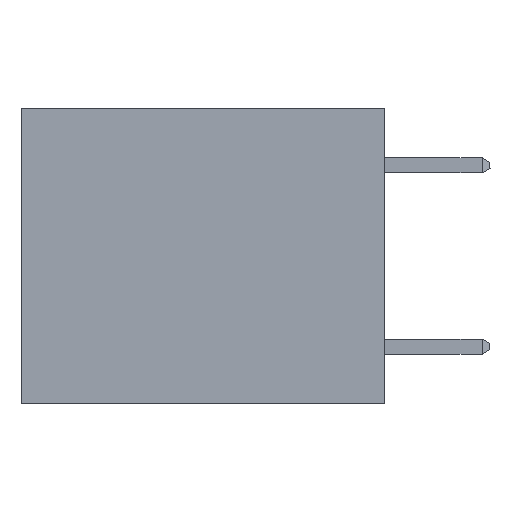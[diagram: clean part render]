
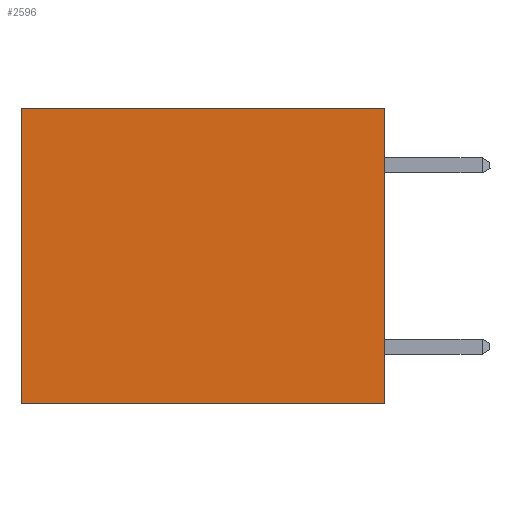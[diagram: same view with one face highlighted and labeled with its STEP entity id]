
A CAD part, left-side view. The second image highlights one B-rep face of the part: STEP entity #2596.
In plain terms, the highlighted planar face has unit normal (-1, 0, 0).
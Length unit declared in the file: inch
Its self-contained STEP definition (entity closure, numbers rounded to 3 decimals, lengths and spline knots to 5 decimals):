
#503 = LINE ( 'NONE', #11311, #14842 ) ;
#2243 = EDGE_LOOP ( 'NONE', ( #10357, #7901, #16710, #20485 ) ) ;
#2596 = ADVANCED_FACE ( 'NONE', ( #7698 ), #6340, .F. ) ;
#2666 = VERTEX_POINT ( 'NONE', #19860 ) ;
#2675 = DIRECTION ( 'NONE',  ( 1., 0., 0. ) ) ;
#3147 = LINE ( 'NONE', #20656, #10557 ) ;
#4397 = LINE ( 'NONE', #13259, #13027 ) ;
#4761 = EDGE_CURVE ( 'NONE', #2666, #6212, #4397, .T. ) ;
#5041 = CARTESIAN_POINT ( 'NONE',  ( 0.3165, 0.6, -0.49 ) ) ;
#6212 = VERTEX_POINT ( 'NONE', #5041 ) ;
#6340 = PLANE ( 'NONE',  #24676 ) ;
#7698 = FACE_OUTER_BOUND ( 'NONE', #2243, .T. ) ;
#7901 = ORIENTED_EDGE ( 'NONE', *, *, #15280, .F. ) ;
#8558 = VERTEX_POINT ( 'NONE', #13615 ) ;
#9403 = DIRECTION ( 'NONE',  ( 0., 0., -1. ) ) ;
#9563 = CARTESIAN_POINT ( 'NONE',  ( 0.3165, 0., -0.49 ) ) ;
#10130 = CARTESIAN_POINT ( 'NONE',  ( 0.3165, 0., -0.49 ) ) ;
#10357 = ORIENTED_EDGE ( 'NONE', *, *, #4761, .T. ) ;
#10557 = VECTOR ( 'NONE', #14275, 39.37008 ) ;
#11311 = CARTESIAN_POINT ( 'NONE',  ( 0.3165, 0., 0. ) ) ;
#11955 = EDGE_CURVE ( 'NONE', #8558, #18296, #21209, .T. ) ;
#12585 = CARTESIAN_POINT ( 'NONE',  ( 0.3165, 0., -0.49 ) ) ;
#13027 = VECTOR ( 'NONE', #23129, 39.37008 ) ;
#13259 = CARTESIAN_POINT ( 'NONE',  ( 0.3165, 0.6, -0.49 ) ) ;
#13426 = EDGE_CURVE ( 'NONE', #8558, #2666, #503, .T. ) ;
#13543 = DIRECTION ( 'NONE',  ( 0., 1., 0. ) ) ;
#13615 = CARTESIAN_POINT ( 'NONE',  ( 0.3165, 0., 0. ) ) ;
#14275 = DIRECTION ( 'NONE',  ( 0., 1., 0. ) ) ;
#14842 = VECTOR ( 'NONE', #13543, 39.37008 ) ;
#15280 = EDGE_CURVE ( 'NONE', #18296, #6212, #3147, .T. ) ;
#16104 = VECTOR ( 'NONE', #9403, 39.37008 ) ;
#16710 = ORIENTED_EDGE ( 'NONE', *, *, #11955, .F. ) ;
#18296 = VERTEX_POINT ( 'NONE', #12585 ) ;
#19860 = CARTESIAN_POINT ( 'NONE',  ( 0.3165, 0.6, 0. ) ) ;
#20485 = ORIENTED_EDGE ( 'NONE', *, *, #13426, .T. ) ;
#20656 = CARTESIAN_POINT ( 'NONE',  ( 0.3165, 0., -0.49 ) ) ;
#21209 = LINE ( 'NONE', #9563, #16104 ) ;
#23129 = DIRECTION ( 'NONE',  ( 0., 0., -1. ) ) ;
#23551 = DIRECTION ( 'NONE',  ( 0., 0., -1. ) ) ;
#24676 = AXIS2_PLACEMENT_3D ( 'NONE', #10130, #2675, #23551 ) ;
